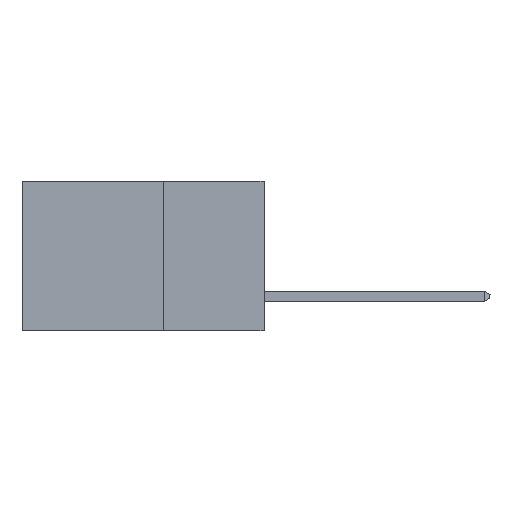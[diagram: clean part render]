
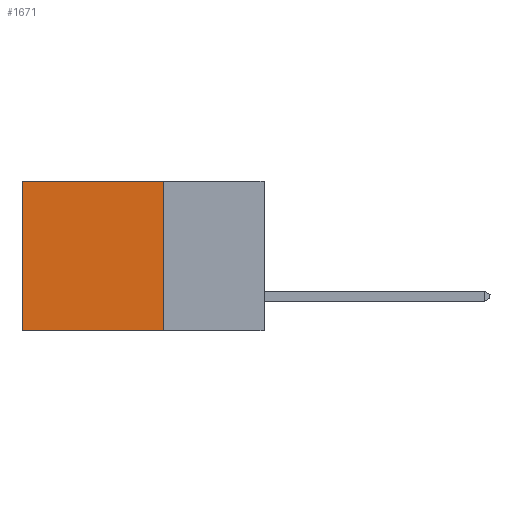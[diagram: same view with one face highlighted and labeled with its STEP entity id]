
A CAD part, left-side view. The second image highlights one B-rep face of the part: STEP entity #1671.
In plain terms, the highlighted planar face has unit normal (-1, 0, 0).
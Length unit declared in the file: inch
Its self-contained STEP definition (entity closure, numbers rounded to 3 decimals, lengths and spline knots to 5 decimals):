
#371 = VERTEX_POINT ( 'NONE', #854 ) ;
#854 = CARTESIAN_POINT ( 'NONE',  ( 0.2615, 0.6, -0.37 ) ) ;
#879 = DIRECTION ( 'NONE',  ( 0., 0., -1. ) ) ;
#957 = VERTEX_POINT ( 'NONE', #11253 ) ;
#1605 = EDGE_CURVE ( 'NONE', #8888, #371, #9757, .T. ) ;
#1671 = ADVANCED_FACE ( 'NONE', ( #5333 ), #8871, .F. ) ;
#2019 = CARTESIAN_POINT ( 'NONE',  ( 0.2615, 0.25, -0.37 ) ) ;
#2852 = CARTESIAN_POINT ( 'NONE',  ( 0.2615, 0.25, 0. ) ) ;
#3077 = CARTESIAN_POINT ( 'NONE',  ( 0.2615, 0.25, 0. ) ) ;
#3441 = ORIENTED_EDGE ( 'NONE', *, *, #1605, .F. ) ;
#3528 = LINE ( 'NONE', #2852, #9259 ) ;
#5333 = FACE_OUTER_BOUND ( 'NONE', #11094, .T. ) ;
#5453 = VECTOR ( 'NONE', #8159, 39.37008 ) ;
#7373 = AXIS2_PLACEMENT_3D ( 'NONE', #2019, #13330, #13248 ) ;
#8151 = CARTESIAN_POINT ( 'NONE',  ( 0.2615, 0.25, -0.37 ) ) ;
#8159 = DIRECTION ( 'NONE',  ( 0., 0., -1. ) ) ;
#8335 = VERTEX_POINT ( 'NONE', #3077 ) ;
#8371 = DIRECTION ( 'NONE',  ( 0., 1., 0. ) ) ;
#8380 = CARTESIAN_POINT ( 'NONE',  ( 0.2615, 0.6, -0.37 ) ) ;
#8840 = ORIENTED_EDGE ( 'NONE', *, *, #13380, .T. ) ;
#8871 = PLANE ( 'NONE',  #7373 ) ;
#8888 = VERTEX_POINT ( 'NONE', #8151 ) ;
#8988 = ORIENTED_EDGE ( 'NONE', *, *, #11206, .T. ) ;
#9259 = VECTOR ( 'NONE', #14180, 39.37008 ) ;
#9285 = VECTOR ( 'NONE', #879, 39.37008 ) ;
#9757 = LINE ( 'NONE', #12884, #10409 ) ;
#10409 = VECTOR ( 'NONE', #8371, 39.37008 ) ;
#10506 = LINE ( 'NONE', #8380, #5453 ) ;
#11081 = CARTESIAN_POINT ( 'NONE',  ( 0.2615, 0.25, -0.37 ) ) ;
#11094 = EDGE_LOOP ( 'NONE', ( #8988, #3441, #11233, #8840 ) ) ;
#11206 = EDGE_CURVE ( 'NONE', #957, #371, #10506, .T. ) ;
#11233 = ORIENTED_EDGE ( 'NONE', *, *, #14524, .F. ) ;
#11253 = CARTESIAN_POINT ( 'NONE',  ( 0.2615, 0.6, 0. ) ) ;
#12356 = LINE ( 'NONE', #11081, #9285 ) ;
#12884 = CARTESIAN_POINT ( 'NONE',  ( 0.2615, 0.25, -0.37 ) ) ;
#13248 = DIRECTION ( 'NONE',  ( 0., 0., -1. ) ) ;
#13330 = DIRECTION ( 'NONE',  ( 1., 0., 0. ) ) ;
#13380 = EDGE_CURVE ( 'NONE', #8335, #957, #3528, .T. ) ;
#14180 = DIRECTION ( 'NONE',  ( 0., 1., 0. ) ) ;
#14524 = EDGE_CURVE ( 'NONE', #8335, #8888, #12356, .T. ) ;
